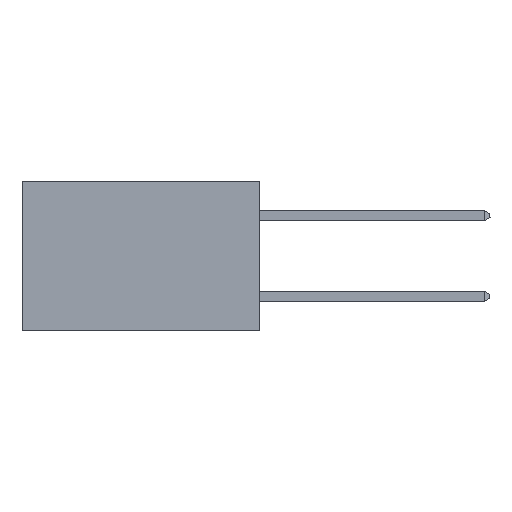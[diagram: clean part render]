
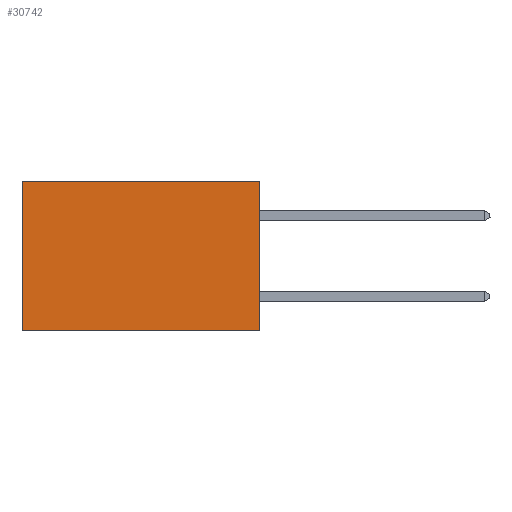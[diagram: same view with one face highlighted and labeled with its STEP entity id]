
A CAD part, left-side view. The second image highlights one B-rep face of the part: STEP entity #30742.
In plain terms, the highlighted planar face has unit normal (-1, 0, 0).
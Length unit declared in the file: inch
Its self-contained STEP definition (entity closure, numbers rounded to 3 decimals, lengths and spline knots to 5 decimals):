
#1343 = VERTEX_POINT ( 'NONE', #19444 ) ;
#2401 = EDGE_CURVE ( 'NONE', #16531, #4138, #33649, .T. ) ;
#4138 = VERTEX_POINT ( 'NONE', #29388 ) ;
#6017 = VECTOR ( 'NONE', #21326, 39.37008 ) ;
#6315 = LINE ( 'NONE', #23751, #19663 ) ;
#6542 = CARTESIAN_POINT ( 'NONE',  ( 0.277, 0.59, 0. ) ) ;
#6941 = FACE_OUTER_BOUND ( 'NONE', #13527, .T. ) ;
#9599 = PLANE ( 'NONE',  #15210 ) ;
#10927 = ORIENTED_EDGE ( 'NONE', *, *, #24185, .F. ) ;
#11822 = DIRECTION ( 'NONE',  ( 0., 0., -1. ) ) ;
#11942 = CARTESIAN_POINT ( 'NONE',  ( 0.277, 0., -0.37 ) ) ;
#13527 = EDGE_LOOP ( 'NONE', ( #20525, #16148, #10927, #25464 ) ) ;
#14994 = DIRECTION ( 'NONE',  ( 0., 0., -1. ) ) ;
#15210 = AXIS2_PLACEMENT_3D ( 'NONE', #27911, #30410, #14994 ) ;
#16148 = ORIENTED_EDGE ( 'NONE', *, *, #2401, .F. ) ;
#16531 = VERTEX_POINT ( 'NONE', #11942 ) ;
#17987 = VERTEX_POINT ( 'NONE', #6542 ) ;
#19444 = CARTESIAN_POINT ( 'NONE',  ( 0.277, 0., 0. ) ) ;
#19663 = VECTOR ( 'NONE', #28843, 39.37008 ) ;
#19721 = CARTESIAN_POINT ( 'NONE',  ( 0.277, 0.59, -0.37 ) ) ;
#19866 = EDGE_CURVE ( 'NONE', #1343, #17987, #32305, .T. ) ;
#20525 = ORIENTED_EDGE ( 'NONE', *, *, #31607, .T. ) ;
#21326 = DIRECTION ( 'NONE',  ( 0., 1., 0. ) ) ;
#23138 = LINE ( 'NONE', #19721, #30163 ) ;
#23284 = CARTESIAN_POINT ( 'NONE',  ( 0.277, 0., -0.37 ) ) ;
#23751 = CARTESIAN_POINT ( 'NONE',  ( 0.277, 0., -0.37 ) ) ;
#24185 = EDGE_CURVE ( 'NONE', #1343, #16531, #6315, .T. ) ;
#25464 = ORIENTED_EDGE ( 'NONE', *, *, #19866, .T. ) ;
#26406 = VECTOR ( 'NONE', #31636, 39.37008 ) ;
#26594 = CARTESIAN_POINT ( 'NONE',  ( 0.277, 0., 0. ) ) ;
#27911 = CARTESIAN_POINT ( 'NONE',  ( 0.277, 0., -0.37 ) ) ;
#28843 = DIRECTION ( 'NONE',  ( 0., 0., -1. ) ) ;
#29388 = CARTESIAN_POINT ( 'NONE',  ( 0.277, 0.59, -0.37 ) ) ;
#30163 = VECTOR ( 'NONE', #11822, 39.37008 ) ;
#30410 = DIRECTION ( 'NONE',  ( 1., 0., 0. ) ) ;
#30742 = ADVANCED_FACE ( 'NONE', ( #6941 ), #9599, .F. ) ;
#31607 = EDGE_CURVE ( 'NONE', #17987, #4138, #23138, .T. ) ;
#31636 = DIRECTION ( 'NONE',  ( 0., 1., 0. ) ) ;
#32305 = LINE ( 'NONE', #26594, #26406 ) ;
#33649 = LINE ( 'NONE', #23284, #6017 ) ;
